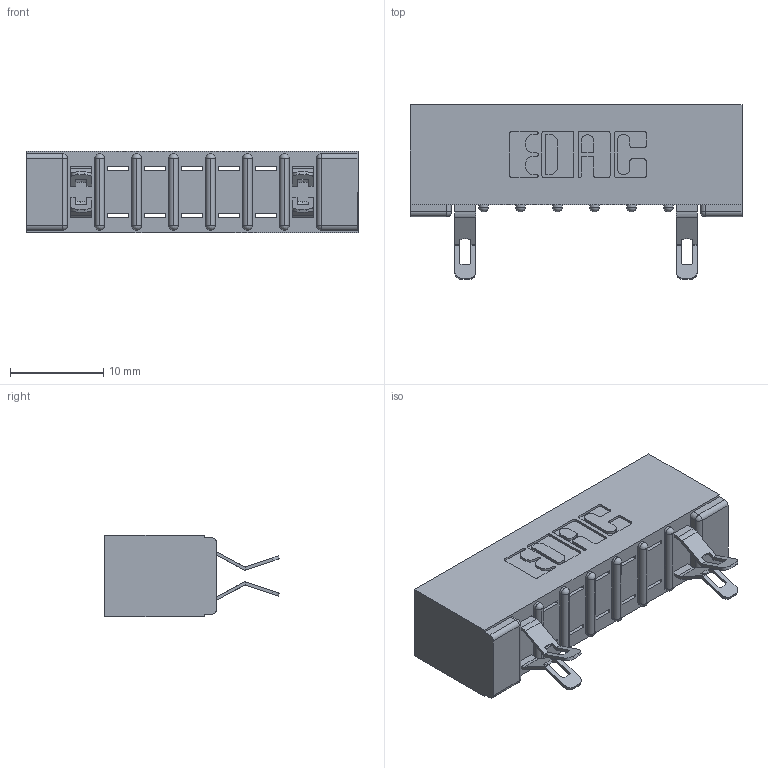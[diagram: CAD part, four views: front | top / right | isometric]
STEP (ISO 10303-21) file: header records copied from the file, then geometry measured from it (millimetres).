
FILE_DESCRIPTION (( 'STEP AP203' ), '1' );
FILE_NAME ('307-014-555-201.STEP', '2018-08-03T01:26:16', ( '' ), ( '' ), 'SwSTEP 2.0', 'SolidWorks 2016', '' );
FILE_SCHEMA (( 'CONFIG_CONTROL_DESIGN' ));
Length unit declared in the file: inch
Products named in the file (3): 307-014-555-201; 307 Part_No Mounting Lugs; 307-290-001_555
Assembly tree (5 placements, depth 2):
  307-014-555-201
    307 Part_No Mounting Lugs
    307-290-001_555  x4
Bounding box: 35.61 x 18.75 x 8.71 mm (x, y, z)
Volume: 2446.6 mm3; surface area: 3310.9 mm2
Topology: 5 solids, 5 shells, 462 faces, 1343 edges, 866 vertices
Faces by surface type: plane 262, cylinder 184, sphere 16
Entity records: 10479 total; most frequent: CARTESIAN_POINT 1769, ORIENTED_EDGE 1760, DIRECTION 1744, EDGE_CURVE 880, LINE 650, VECTOR 650, VERTEX_POINT 572, AXIS2_PLACEMENT_3D 547
